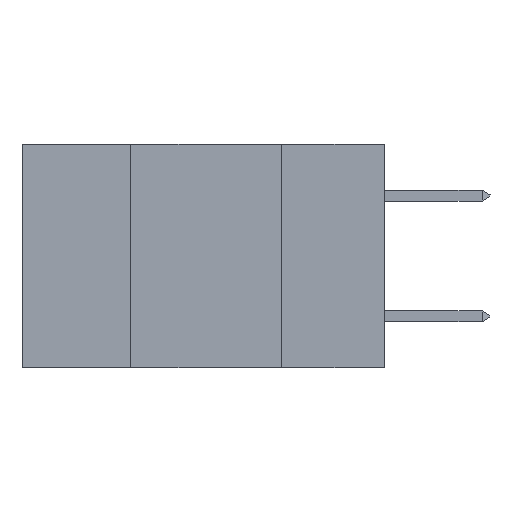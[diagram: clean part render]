
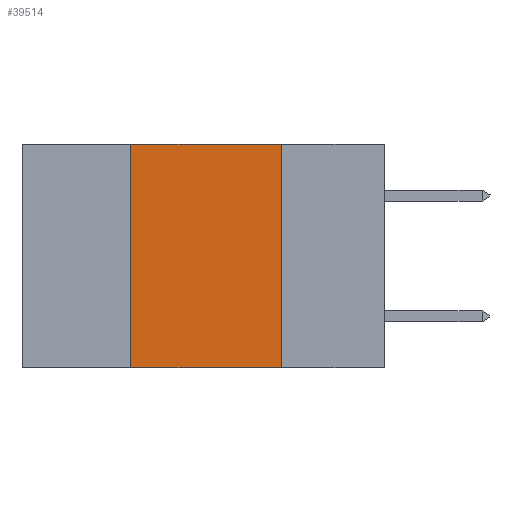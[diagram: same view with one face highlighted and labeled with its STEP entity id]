
A CAD part, left-side view. The second image highlights one B-rep face of the part: STEP entity #39514.
In plain terms, the highlighted planar face has unit normal (-1, 0, 0).
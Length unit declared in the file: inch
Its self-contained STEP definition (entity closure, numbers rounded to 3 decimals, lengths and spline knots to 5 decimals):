
#698 = CARTESIAN_POINT ( 'NONE',  ( 0., 0.42, 0. ) ) ;
#2255 = CARTESIAN_POINT ( 'NONE',  ( 0., 0.17, 0. ) ) ;
#3173 = LINE ( 'NONE', #26939, #15844 ) ;
#4378 = VECTOR ( 'NONE', #36428, 39.37008 ) ;
#4565 = EDGE_CURVE ( 'NONE', #35249, #6893, #35592, .T. ) ;
#4673 = DIRECTION ( 'NONE',  ( 0., 0., -1. ) ) ;
#6893 = VERTEX_POINT ( 'NONE', #21245 ) ;
#7021 = ORIENTED_EDGE ( 'NONE', *, *, #35157, .F. ) ;
#7678 = PLANE ( 'NONE',  #32930 ) ;
#7781 = EDGE_LOOP ( 'NONE', ( #9967, #7021, #20865, #38043 ) ) ;
#9967 = ORIENTED_EDGE ( 'NONE', *, *, #22816, .F. ) ;
#15844 = VECTOR ( 'NONE', #33182, 39.37008 ) ;
#17173 = LINE ( 'NONE', #30890, #20089 ) ;
#17581 = CARTESIAN_POINT ( 'NONE',  ( 0., 0.6, -0.37 ) ) ;
#20089 = VECTOR ( 'NONE', #24771, 39.37008 ) ;
#20865 = ORIENTED_EDGE ( 'NONE', *, *, #26155, .F. ) ;
#21245 = CARTESIAN_POINT ( 'NONE',  ( 0., 0.17, -0.37 ) ) ;
#22816 = EDGE_CURVE ( 'NONE', #36864, #6893, #24850, .T. ) ;
#24771 = DIRECTION ( 'NONE',  ( 0., -1., 0. ) ) ;
#24850 = LINE ( 'NONE', #2255, #4378 ) ;
#26155 = EDGE_CURVE ( 'NONE', #35249, #27126, #3173, .T. ) ;
#26697 = DIRECTION ( 'NONE',  ( 0., -1., 0. ) ) ;
#26939 = CARTESIAN_POINT ( 'NONE',  ( 0., 0.42, 0. ) ) ;
#27126 = VERTEX_POINT ( 'NONE', #698 ) ;
#29464 = DIRECTION ( 'NONE',  ( 1., 0., 0. ) ) ;
#29518 = CARTESIAN_POINT ( 'NONE',  ( 0., 0.17, 0. ) ) ;
#30890 = CARTESIAN_POINT ( 'NONE',  ( 0., 0.6, 0. ) ) ;
#31431 = FACE_OUTER_BOUND ( 'NONE', #7781, .T. ) ;
#31660 = VECTOR ( 'NONE', #26697, 39.37008 ) ;
#32930 = AXIS2_PLACEMENT_3D ( 'NONE', #38613, #29464, #4673 ) ;
#33182 = DIRECTION ( 'NONE',  ( 0., 0., 1. ) ) ;
#35157 = EDGE_CURVE ( 'NONE', #27126, #36864, #17173, .T. ) ;
#35249 = VERTEX_POINT ( 'NONE', #37238 ) ;
#35592 = LINE ( 'NONE', #17581, #31660 ) ;
#36428 = DIRECTION ( 'NONE',  ( 0., 0., -1. ) ) ;
#36864 = VERTEX_POINT ( 'NONE', #29518 ) ;
#37238 = CARTESIAN_POINT ( 'NONE',  ( 0., 0.42, -0.37 ) ) ;
#38043 = ORIENTED_EDGE ( 'NONE', *, *, #4565, .T. ) ;
#38613 = CARTESIAN_POINT ( 'NONE',  ( 0., 0.6, 0. ) ) ;
#39514 = ADVANCED_FACE ( 'NONE', ( #31431 ), #7678, .F. ) ;
